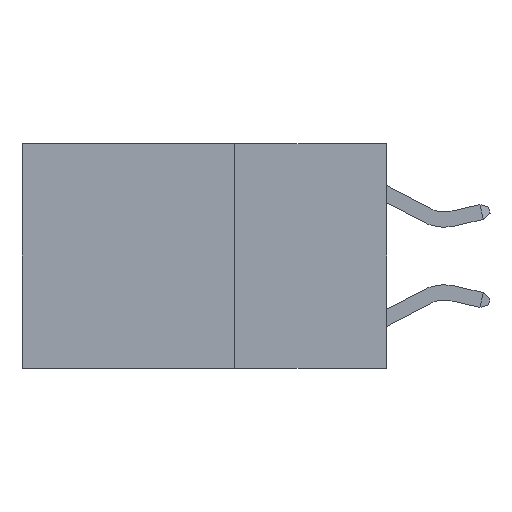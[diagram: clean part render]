
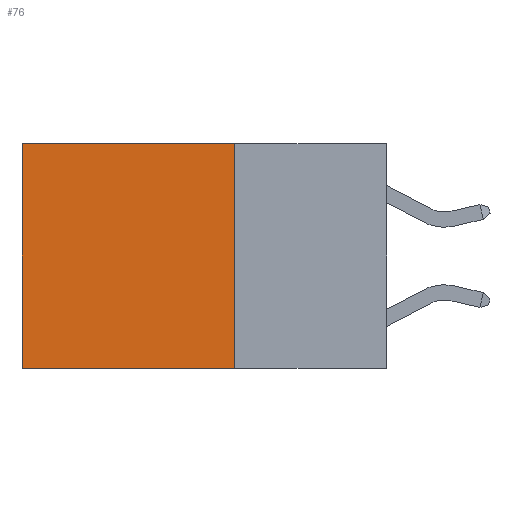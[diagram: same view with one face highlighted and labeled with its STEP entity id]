
A CAD part, left-side view. The second image highlights one B-rep face of the part: STEP entity #76.
In plain terms, the highlighted planar face has unit normal (-1, 0, 0).
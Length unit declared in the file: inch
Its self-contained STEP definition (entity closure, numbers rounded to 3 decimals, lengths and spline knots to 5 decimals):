
#76 = ADVANCED_FACE ( 'NONE', ( #4096 ), #9578, .F. ) ;
#279 = CARTESIAN_POINT ( 'NONE',  ( 0.2625, 0.25, -0.37 ) ) ;
#285 = VECTOR ( 'NONE', #413, 39.37008 ) ;
#413 = DIRECTION ( 'NONE',  ( 0., 0., -1. ) ) ;
#1536 = DIRECTION ( 'NONE',  ( 0., 0., -1. ) ) ;
#1666 = CARTESIAN_POINT ( 'NONE',  ( 0.2625, 0.25, 0. ) ) ;
#3507 = CARTESIAN_POINT ( 'NONE',  ( 0.2625, 0.6, 0. ) ) ;
#3537 = ORIENTED_EDGE ( 'NONE', *, *, #8162, .T. ) ;
#3557 = CARTESIAN_POINT ( 'NONE',  ( 0.2625, 0.25, 0. ) ) ;
#3700 = CARTESIAN_POINT ( 'NONE',  ( 0.2625, 0.25, -0.37 ) ) ;
#3861 = ORIENTED_EDGE ( 'NONE', *, *, #7753, .T. ) ;
#4096 = FACE_OUTER_BOUND ( 'NONE', #7634, .T. ) ;
#4336 = VECTOR ( 'NONE', #1536, 39.37008 ) ;
#4985 = CARTESIAN_POINT ( 'NONE',  ( 0.2625, 0.6, -0.37 ) ) ;
#5069 = EDGE_CURVE ( 'NONE', #7004, #8927, #9898, .T. ) ;
#5393 = CARTESIAN_POINT ( 'NONE',  ( 0.2625, 0.25, 0. ) ) ;
#5724 = LINE ( 'NONE', #8904, #4336 ) ;
#5764 = VERTEX_POINT ( 'NONE', #3557 ) ;
#6066 = ORIENTED_EDGE ( 'NONE', *, *, #6834, .F. ) ;
#6708 = VECTOR ( 'NONE', #8567, 39.37008 ) ;
#6834 = EDGE_CURVE ( 'NONE', #5764, #7004, #5724, .T. ) ;
#6964 = LINE ( 'NONE', #7666, #285 ) ;
#7004 = VERTEX_POINT ( 'NONE', #279 ) ;
#7282 = DIRECTION ( 'NONE',  ( 1., 0., 0. ) ) ;
#7320 = DIRECTION ( 'NONE',  ( 0., 0., -1. ) ) ;
#7525 = VECTOR ( 'NONE', #7676, 39.37008 ) ;
#7634 = EDGE_LOOP ( 'NONE', ( #3537, #9427, #6066, #3861 ) ) ;
#7666 = CARTESIAN_POINT ( 'NONE',  ( 0.2625, 0.6, 0. ) ) ;
#7676 = DIRECTION ( 'NONE',  ( 0., 1., 0. ) ) ;
#7753 = EDGE_CURVE ( 'NONE', #5764, #9754, #8619, .T. ) ;
#8162 = EDGE_CURVE ( 'NONE', #9754, #8927, #6964, .T. ) ;
#8567 = DIRECTION ( 'NONE',  ( 0., 1., 0. ) ) ;
#8619 = LINE ( 'NONE', #5393, #6708 ) ;
#8904 = CARTESIAN_POINT ( 'NONE',  ( 0.2625, 0.25, 0. ) ) ;
#8927 = VERTEX_POINT ( 'NONE', #4985 ) ;
#9427 = ORIENTED_EDGE ( 'NONE', *, *, #5069, .F. ) ;
#9578 = PLANE ( 'NONE',  #10108 ) ;
#9754 = VERTEX_POINT ( 'NONE', #3507 ) ;
#9898 = LINE ( 'NONE', #3700, #7525 ) ;
#10108 = AXIS2_PLACEMENT_3D ( 'NONE', #1666, #7282, #7320 ) ;
